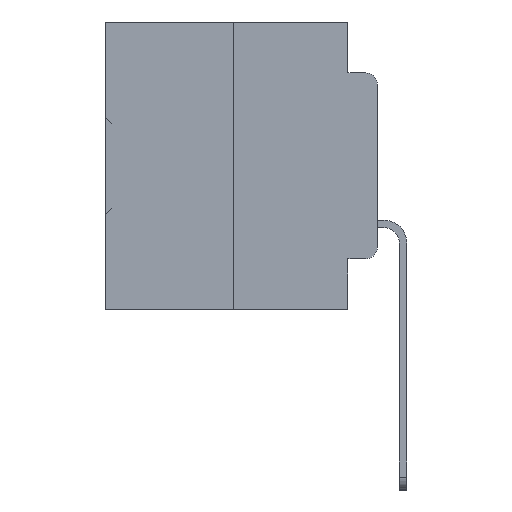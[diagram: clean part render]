
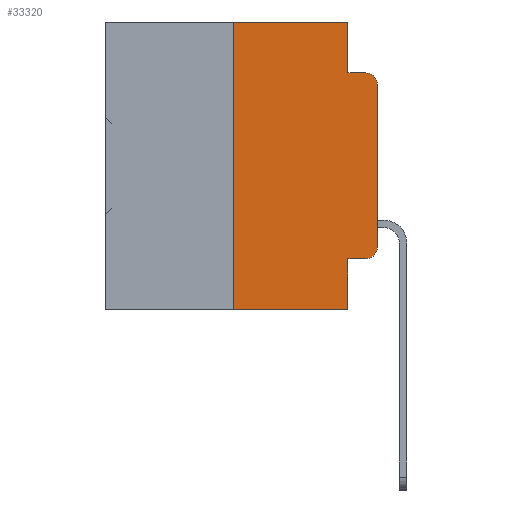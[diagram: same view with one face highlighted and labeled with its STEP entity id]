
A CAD part, left-side view. The second image highlights one B-rep face of the part: STEP entity #33320.
In plain terms, the highlighted planar face has unit normal (-1, 0, 0).
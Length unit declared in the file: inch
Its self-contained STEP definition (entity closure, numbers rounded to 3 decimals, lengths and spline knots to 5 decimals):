
#121 = CARTESIAN_POINT ( 'NONE',  ( 0., 0.051, -0.5 ) ) ;
#380 = CARTESIAN_POINT ( 'NONE',  ( 0., 0.473, -0.5 ) ) ;
#1380 = CARTESIAN_POINT ( 'NONE',  ( 0., 0.051, -0.4115 ) ) ;
#1384 = DIRECTION ( 'NONE',  ( 0., 0., -1. ) ) ;
#2825 = DIRECTION ( 'NONE',  ( 0., 0., -1. ) ) ;
#3032 = CARTESIAN_POINT ( 'NONE',  ( 0., 0., -0.3915 ) ) ;
#3244 = VECTOR ( 'NONE', #35560, 39.37008 ) ;
#3479 = DIRECTION ( 'NONE',  ( 0., -1., 0. ) ) ;
#3530 = VERTEX_POINT ( 'NONE', #9776 ) ;
#3603 = DIRECTION ( 'NONE',  ( 0., 0., -1. ) ) ;
#4008 = CARTESIAN_POINT ( 'NONE',  ( 0., 0.051, -0.0885 ) ) ;
#4239 = DIRECTION ( 'NONE',  ( 0., -1., 0. ) ) ;
#4732 = VERTEX_POINT ( 'NONE', #13966 ) ;
#4867 = ORIENTED_EDGE ( 'NONE', *, *, #14339, .T. ) ;
#5201 = DIRECTION ( 'NONE',  ( 0., 0., -1. ) ) ;
#5907 = EDGE_CURVE ( 'NONE', #8359, #14071, #36073, .T. ) ;
#6172 = LINE ( 'NONE', #29796, #20009 ) ;
#6932 = VERTEX_POINT ( 'NONE', #10186 ) ;
#7330 = VECTOR ( 'NONE', #4239, 39.37008 ) ;
#8211 = CARTESIAN_POINT ( 'NONE',  ( 0., 0.25, -0.5 ) ) ;
#8359 = VERTEX_POINT ( 'NONE', #1380 ) ;
#8837 = VECTOR ( 'NONE', #3479, 39.37008 ) ;
#9170 = LINE ( 'NONE', #36675, #7330 ) ;
#9776 = CARTESIAN_POINT ( 'NONE',  ( 0., 0.25, 0. ) ) ;
#10011 = AXIS2_PLACEMENT_3D ( 'NONE', #32661, #14955, #2825 ) ;
#10186 = CARTESIAN_POINT ( 'NONE',  ( 0., 0.051, 0. ) ) ;
#10412 = CARTESIAN_POINT ( 'NONE',  ( 0., 0.02, -0.4115 ) ) ;
#10465 = EDGE_CURVE ( 'NONE', #35328, #27610, #6172, .T. ) ;
#10646 = ORIENTED_EDGE ( 'NONE', *, *, #27108, .F. ) ;
#10815 = VECTOR ( 'NONE', #3603, 39.37008 ) ;
#10860 = CARTESIAN_POINT ( 'NONE',  ( 0., 0.473, 0. ) ) ;
#12635 = DIRECTION ( 'NONE',  ( 1., 0., 0. ) ) ;
#13001 = CARTESIAN_POINT ( 'NONE',  ( 0., 0.02, -0.0885 ) ) ;
#13966 = CARTESIAN_POINT ( 'NONE',  ( 0., 0., -0.1085 ) ) ;
#14071 = VERTEX_POINT ( 'NONE', #121 ) ;
#14339 = EDGE_CURVE ( 'NONE', #8359, #20648, #9170, .T. ) ;
#14464 = ORIENTED_EDGE ( 'NONE', *, *, #21669, .T. ) ;
#14876 = EDGE_LOOP ( 'NONE', ( #23902, #36506, #21704, #31447, #10646, #32586, #14464, #34498, #4867, #20244 ) ) ;
#14955 = DIRECTION ( 'NONE',  ( -1., 0., 0. ) ) ;
#15140 = DIRECTION ( 'NONE',  ( 0., 0., 1. ) ) ;
#15241 = CARTESIAN_POINT ( 'NONE',  ( 0., 0.051, 0. ) ) ;
#16542 = LINE ( 'NONE', #10860, #31783 ) ;
#16701 = CARTESIAN_POINT ( 'NONE',  ( 0., 0., 0. ) ) ;
#16915 = AXIS2_PLACEMENT_3D ( 'NONE', #25742, #28718, #5201 ) ;
#17736 = LINE ( 'NONE', #15241, #10815 ) ;
#18475 = CIRCLE ( 'NONE', #16915, 0.02 ) ;
#19119 = VERTEX_POINT ( 'NONE', #3032 ) ;
#19162 = CIRCLE ( 'NONE', #10011, 0.02 ) ;
#19506 = EDGE_CURVE ( 'NONE', #19119, #4732, #23313, .T. ) ;
#19802 = EDGE_CURVE ( 'NONE', #6932, #35328, #17736, .T. ) ;
#20009 = VECTOR ( 'NONE', #35472, 39.37008 ) ;
#20244 = ORIENTED_EDGE ( 'NONE', *, *, #38288, .T. ) ;
#20648 = VERTEX_POINT ( 'NONE', #10412 ) ;
#20716 = LINE ( 'NONE', #29760, #35513 ) ;
#20967 = AXIS2_PLACEMENT_3D ( 'NONE', #30732, #12635, #1384 ) ;
#21291 = PLANE ( 'NONE',  #20967 ) ;
#21669 = EDGE_CURVE ( 'NONE', #37365, #14071, #29197, .T. ) ;
#21704 = ORIENTED_EDGE ( 'NONE', *, *, #10465, .F. ) ;
#22645 = DIRECTION ( 'NONE',  ( 0., 0., 1. ) ) ;
#23313 = LINE ( 'NONE', #16701, #36269 ) ;
#23902 = ORIENTED_EDGE ( 'NONE', *, *, #19506, .T. ) ;
#25742 = CARTESIAN_POINT ( 'NONE',  ( 0., 0.02, -0.3915 ) ) ;
#27108 = EDGE_CURVE ( 'NONE', #3530, #6932, #16542, .T. ) ;
#27610 = VERTEX_POINT ( 'NONE', #13001 ) ;
#28718 = DIRECTION ( 'NONE',  ( -1., 0., 0. ) ) ;
#29197 = LINE ( 'NONE', #380, #8837 ) ;
#29502 = EDGE_CURVE ( 'NONE', #4732, #27610, #19162, .T. ) ;
#29760 = CARTESIAN_POINT ( 'NONE',  ( 0., 0.25, 0. ) ) ;
#29796 = CARTESIAN_POINT ( 'NONE',  ( 0., 0.051, -0.0885 ) ) ;
#30732 = CARTESIAN_POINT ( 'NONE',  ( 0., 0.473, 0. ) ) ;
#31447 = ORIENTED_EDGE ( 'NONE', *, *, #19802, .F. ) ;
#31647 = DIRECTION ( 'NONE',  ( 0., -1., 0. ) ) ;
#31783 = VECTOR ( 'NONE', #31647, 39.37008 ) ;
#32335 = FACE_OUTER_BOUND ( 'NONE', #14876, .T. ) ;
#32586 = ORIENTED_EDGE ( 'NONE', *, *, #34261, .F. ) ;
#32661 = CARTESIAN_POINT ( 'NONE',  ( 0., 0.02, -0.1085 ) ) ;
#33320 = ADVANCED_FACE ( 'NONE', ( #32335 ), #21291, .F. ) ;
#34261 = EDGE_CURVE ( 'NONE', #37365, #3530, #20716, .T. ) ;
#34498 = ORIENTED_EDGE ( 'NONE', *, *, #5907, .F. ) ;
#35328 = VERTEX_POINT ( 'NONE', #4008 ) ;
#35472 = DIRECTION ( 'NONE',  ( 0., -1., 0. ) ) ;
#35513 = VECTOR ( 'NONE', #15140, 39.37008 ) ;
#35560 = DIRECTION ( 'NONE',  ( 0., 0., -1. ) ) ;
#35808 = CARTESIAN_POINT ( 'NONE',  ( 0., 0.051, 0. ) ) ;
#36073 = LINE ( 'NONE', #35808, #3244 ) ;
#36269 = VECTOR ( 'NONE', #22645, 39.37008 ) ;
#36506 = ORIENTED_EDGE ( 'NONE', *, *, #29502, .T. ) ;
#36675 = CARTESIAN_POINT ( 'NONE',  ( 0., 0.051, -0.4115 ) ) ;
#37365 = VERTEX_POINT ( 'NONE', #8211 ) ;
#38288 = EDGE_CURVE ( 'NONE', #20648, #19119, #18475, .T. ) ;
